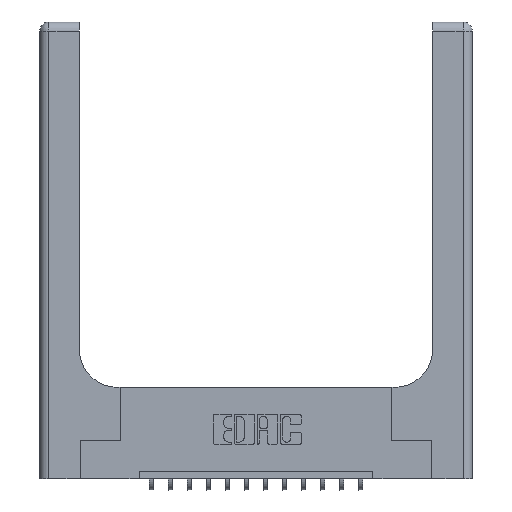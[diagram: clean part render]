
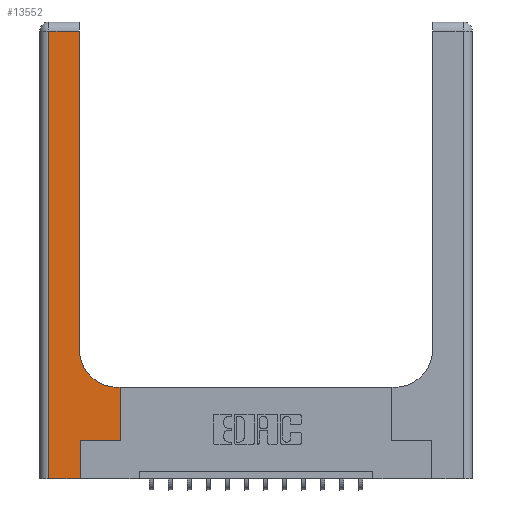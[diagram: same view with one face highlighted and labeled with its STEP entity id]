
A CAD part, top view. The second image highlights one B-rep face of the part: STEP entity #13552.
In plain terms, the highlighted planar face has unit normal (0, 0, 1).
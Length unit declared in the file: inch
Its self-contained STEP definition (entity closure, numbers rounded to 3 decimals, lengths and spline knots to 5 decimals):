
#80 = LINE ( 'NONE', #12507, #6610 ) ;
#154 = VERTEX_POINT ( 'NONE', #6922 ) ;
#178 = VERTEX_POINT ( 'NONE', #1877 ) ;
#567 = DIRECTION ( 'NONE',  ( 0., 1., 0. ) ) ;
#587 = LINE ( 'NONE', #8965, #7498 ) ;
#1056 = AXIS2_PLACEMENT_3D ( 'NONE', #8974, #1272, #10315 ) ;
#1260 = DIRECTION ( 'NONE',  ( 1., 0., 0. ) ) ;
#1272 = DIRECTION ( 'NONE',  ( 0., 0., -1. ) ) ;
#1750 = ORIENTED_EDGE ( 'NONE', *, *, #5066, .T. ) ;
#1877 = CARTESIAN_POINT ( 'NONE',  ( 0.06, 2.94, 0.37 ) ) ;
#1882 = EDGE_CURVE ( 'NONE', #15413, #16594, #15909, .T. ) ;
#1913 = LINE ( 'NONE', #9801, #8748 ) ;
#2225 = EDGE_LOOP ( 'NONE', ( #1750, #8997, #15903, #16314, #6431, #16695, #8020, #11897, #15323 ) ) ;
#2287 = EDGE_CURVE ( 'NONE', #16594, #154, #9830, .T. ) ;
#2468 = CARTESIAN_POINT ( 'NONE',  ( 0.06, 3., 0.37 ) ) ;
#2726 = DIRECTION ( 'NONE',  ( -1., 0., 0. ) ) ;
#2931 = CARTESIAN_POINT ( 'NONE',  ( 0.528, 0.6, 0.37 ) ) ;
#2943 = CIRCLE ( 'NONE', #1056, 0.25 ) ;
#3117 = CARTESIAN_POINT ( 'NONE',  ( 0., 3., 0.37 ) ) ;
#3493 = EDGE_CURVE ( 'NONE', #13550, #14252, #14766, .T. ) ;
#3530 = FACE_OUTER_BOUND ( 'NONE', #2225, .T. ) ;
#3641 = CARTESIAN_POINT ( 'NONE',  ( 0., 0., 0.37 ) ) ;
#3718 = VERTEX_POINT ( 'NONE', #4769 ) ;
#3746 = DIRECTION ( 'NONE',  ( 0., -1., 0. ) ) ;
#4381 = DIRECTION ( 'NONE',  ( -1., 0., 0. ) ) ;
#4769 = CARTESIAN_POINT ( 'NONE',  ( 0.26, 0.85, 0.37 ) ) ;
#4945 = DIRECTION ( 'NONE',  ( 1., 0., 0. ) ) ;
#5066 = EDGE_CURVE ( 'NONE', #3718, #8104, #80, .T. ) ;
#6223 = EDGE_CURVE ( 'NONE', #8104, #178, #1913, .T. ) ;
#6377 = EDGE_CURVE ( 'NONE', #178, #15413, #16643, .T. ) ;
#6400 = EDGE_CURVE ( 'NONE', #8297, #3718, #2943, .T. ) ;
#6431 = ORIENTED_EDGE ( 'NONE', *, *, #2287, .T. ) ;
#6610 = VECTOR ( 'NONE', #11161, 39.37008 ) ;
#6889 = CARTESIAN_POINT ( 'NONE',  ( 0.528, 0.25, 0.37 ) ) ;
#6922 = CARTESIAN_POINT ( 'NONE',  ( 0.265, 0.25, 0.37 ) ) ;
#6959 = CARTESIAN_POINT ( 'NONE',  ( 0.528, 0.25, 0.37 ) ) ;
#7446 = CARTESIAN_POINT ( 'NONE',  ( 0.265, 0., 0.37 ) ) ;
#7498 = VECTOR ( 'NONE', #1260, 39.37008 ) ;
#7835 = CARTESIAN_POINT ( 'NONE',  ( 0.26, 0.6, 0.37 ) ) ;
#7853 = VECTOR ( 'NONE', #8157, 39.37008 ) ;
#8020 = ORIENTED_EDGE ( 'NONE', *, *, #3493, .T. ) ;
#8104 = VERTEX_POINT ( 'NONE', #11123 ) ;
#8157 = DIRECTION ( 'NONE',  ( 0., 1., 0. ) ) ;
#8297 = VERTEX_POINT ( 'NONE', #8874 ) ;
#8748 = VECTOR ( 'NONE', #11114, 39.37008 ) ;
#8874 = CARTESIAN_POINT ( 'NONE',  ( 0.51, 0.6, 0.37 ) ) ;
#8965 = CARTESIAN_POINT ( 'NONE',  ( 0.265, 0.25, 0.37 ) ) ;
#8974 = CARTESIAN_POINT ( 'NONE',  ( 0.51, 0.85, 0.37 ) ) ;
#8997 = ORIENTED_EDGE ( 'NONE', *, *, #6223, .T. ) ;
#9609 = CARTESIAN_POINT ( 'NONE',  ( 0.265, 0., 0.37 ) ) ;
#9782 = VECTOR ( 'NONE', #3746, 39.37008 ) ;
#9801 = CARTESIAN_POINT ( 'NONE',  ( 0., 2.94, 0.37 ) ) ;
#9830 = LINE ( 'NONE', #9609, #16304 ) ;
#10315 = DIRECTION ( 'NONE',  ( 1., 0., 0. ) ) ;
#10369 = EDGE_CURVE ( 'NONE', #154, #13550, #587, .T. ) ;
#10843 = PLANE ( 'NONE',  #11230 ) ;
#11114 = DIRECTION ( 'NONE',  ( -1., 0., 0. ) ) ;
#11123 = CARTESIAN_POINT ( 'NONE',  ( 0.26, 2.94, 0.37 ) ) ;
#11161 = DIRECTION ( 'NONE',  ( 0., 1., 0. ) ) ;
#11230 = AXIS2_PLACEMENT_3D ( 'NONE', #3117, #12175, #4381 ) ;
#11897 = ORIENTED_EDGE ( 'NONE', *, *, #15420, .T. ) ;
#12175 = DIRECTION ( 'NONE',  ( 0., 0., -1. ) ) ;
#12507 = CARTESIAN_POINT ( 'NONE',  ( 0.26, 3., 0.37 ) ) ;
#12532 = VECTOR ( 'NONE', #4945, 39.37008 ) ;
#13021 = VECTOR ( 'NONE', #2726, 39.37008 ) ;
#13550 = VERTEX_POINT ( 'NONE', #6959 ) ;
#13552 = ADVANCED_FACE ( 'NONE', ( #3530 ), #10843, .F. ) ;
#13818 = LINE ( 'NONE', #7835, #13021 ) ;
#14252 = VERTEX_POINT ( 'NONE', #2931 ) ;
#14766 = LINE ( 'NONE', #6889, #7853 ) ;
#15323 = ORIENTED_EDGE ( 'NONE', *, *, #6400, .T. ) ;
#15413 = VERTEX_POINT ( 'NONE', #15588 ) ;
#15420 = EDGE_CURVE ( 'NONE', #14252, #8297, #13818, .T. ) ;
#15588 = CARTESIAN_POINT ( 'NONE',  ( 0.06, 0., 0.37 ) ) ;
#15903 = ORIENTED_EDGE ( 'NONE', *, *, #6377, .T. ) ;
#15909 = LINE ( 'NONE', #3641, #12532 ) ;
#16304 = VECTOR ( 'NONE', #567, 39.37008 ) ;
#16314 = ORIENTED_EDGE ( 'NONE', *, *, #1882, .T. ) ;
#16594 = VERTEX_POINT ( 'NONE', #7446 ) ;
#16643 = LINE ( 'NONE', #2468, #9782 ) ;
#16695 = ORIENTED_EDGE ( 'NONE', *, *, #10369, .T. ) ;
